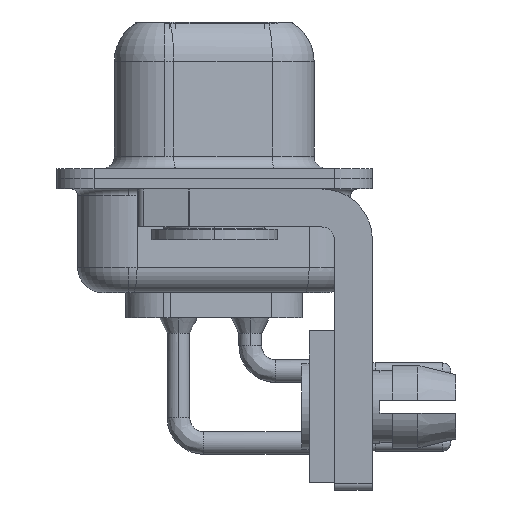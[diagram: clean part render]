
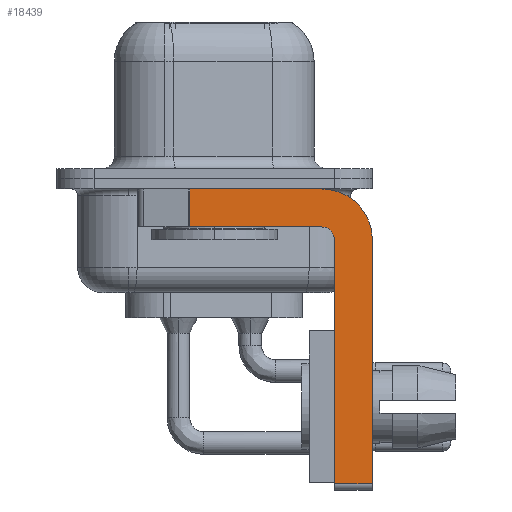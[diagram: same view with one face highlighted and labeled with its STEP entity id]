
A CAD part, left-side view. The second image highlights one B-rep face of the part: STEP entity #18439.
In plain terms, the highlighted planar face has unit normal (-1, 0, 0).
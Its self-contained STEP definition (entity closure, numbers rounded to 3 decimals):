
#227 = EDGE_LOOP ( 'NONE', ( #13423, #16876, #19151, #14804, #31102, #12259, #10388, #13263 ) ) ;
#1313 = LINE ( 'NONE', #20299, #27001 ) ;
#1387 = EDGE_CURVE ( 'NONE', #9785, #28108, #3314, .T. ) ;
#2059 = LINE ( 'NONE', #22127, #14434 ) ;
#2197 = VERTEX_POINT ( 'NONE', #12103 ) ;
#3314 = CIRCLE ( 'NONE', #14173, 2. ) ;
#3638 = VERTEX_POINT ( 'NONE', #23678 ) ;
#3837 = LINE ( 'NONE', #17102, #9616 ) ;
#4691 = DIRECTION ( 'NONE',  ( 0., 0., 1. ) ) ;
#5693 = CARTESIAN_POINT ( 'NONE',  ( -2.9, -4.75, -2.4 ) ) ;
#6016 = DIRECTION ( 'NONE',  ( 0., 0., -1. ) ) ;
#7905 = EDGE_CURVE ( 'NONE', #11101, #25925, #14828, .T. ) ;
#8450 = VECTOR ( 'NONE', #6016, 1000. ) ;
#8511 = VECTOR ( 'NONE', #18971, 1000. ) ;
#8834 = AXIS2_PLACEMENT_3D ( 'NONE', #12398, #29939, #14908 ) ;
#9466 = EDGE_CURVE ( 'NONE', #22974, #2197, #21409, .T. ) ;
#9616 = VECTOR ( 'NONE', #4691, 1000. ) ;
#9785 = VERTEX_POINT ( 'NONE', #25731 ) ;
#10388 = ORIENTED_EDGE ( 'NONE', *, *, #11176, .F. ) ;
#11101 = VERTEX_POINT ( 'NONE', #5693 ) ;
#11176 = EDGE_CURVE ( 'NONE', #28108, #3638, #20982, .T. ) ;
#11508 = CARTESIAN_POINT ( 'NONE',  ( -2.9, -4.25, -12.05 ) ) ;
#12103 = CARTESIAN_POINT ( 'NONE',  ( -2.9, 0.978, -1.9 ) ) ;
#12259 = ORIENTED_EDGE ( 'NONE', *, *, #15803, .T. ) ;
#12398 = CARTESIAN_POINT ( 'NONE',  ( -2.9, -4.25, -2.4 ) ) ;
#12971 = CARTESIAN_POINT ( 'NONE',  ( -2.9, -4.25, -2.4 ) ) ;
#13248 = CARTESIAN_POINT ( 'NONE',  ( -2.9, -4.75, -12.05 ) ) ;
#13263 = ORIENTED_EDGE ( 'NONE', *, *, #1387, .F. ) ;
#13423 = ORIENTED_EDGE ( 'NONE', *, *, #22481, .F. ) ;
#13800 = DIRECTION ( 'NONE',  ( 0., 0., -1. ) ) ;
#14131 = EDGE_CURVE ( 'NONE', #25925, #2197, #1313, .T. ) ;
#14173 = AXIS2_PLACEMENT_3D ( 'NONE', #14402, #14373, #13800 ) ;
#14371 = LINE ( 'NONE', #11508, #8511 ) ;
#14373 = DIRECTION ( 'NONE',  ( 1., 0., 0. ) ) ;
#14402 = CARTESIAN_POINT ( 'NONE',  ( -2.9, -4.25, -2.4 ) ) ;
#14434 = VECTOR ( 'NONE', #22235, 1000. ) ;
#14736 = VECTOR ( 'NONE', #24557, 1000. ) ;
#14804 = ORIENTED_EDGE ( 'NONE', *, *, #7905, .F. ) ;
#14828 = CIRCLE ( 'NONE', #20042, 0.5 ) ;
#14908 = DIRECTION ( 'NONE',  ( 0., 0., -1. ) ) ;
#15203 = CARTESIAN_POINT ( 'NONE',  ( -2.9, -6.25, -2.4 ) ) ;
#15358 = DIRECTION ( 'NONE',  ( 0., 1., 0. ) ) ;
#15482 = DIRECTION ( 'NONE',  ( 0., 0., 1. ) ) ;
#15803 = EDGE_CURVE ( 'NONE', #31345, #3638, #14371, .T. ) ;
#16876 = ORIENTED_EDGE ( 'NONE', *, *, #9466, .T. ) ;
#17018 = CARTESIAN_POINT ( 'NONE',  ( -2.9, 0.978, -1.9 ) ) ;
#17102 = CARTESIAN_POINT ( 'NONE',  ( -2.9, -4.75, -12.3 ) ) ;
#18439 = ADVANCED_FACE ( 'NONE', ( #31940 ), #27383, .F. ) ;
#18971 = DIRECTION ( 'NONE',  ( 0., -1., 0. ) ) ;
#19151 = ORIENTED_EDGE ( 'NONE', *, *, #14131, .F. ) ;
#20042 = AXIS2_PLACEMENT_3D ( 'NONE', #12971, #30501, #15482 ) ;
#20299 = CARTESIAN_POINT ( 'NONE',  ( -2.9, -4.25, -1.9 ) ) ;
#20962 = CARTESIAN_POINT ( 'NONE',  ( -2.9, -6.25, -2.4 ) ) ;
#20982 = LINE ( 'NONE', #20962, #8450 ) ;
#21409 = LINE ( 'NONE', #17018, #14736 ) ;
#22127 = CARTESIAN_POINT ( 'NONE',  ( -2.9, 3., -0.4 ) ) ;
#22235 = DIRECTION ( 'NONE',  ( 0., -1., 0. ) ) ;
#22481 = EDGE_CURVE ( 'NONE', #22974, #9785, #2059, .T. ) ;
#22974 = VERTEX_POINT ( 'NONE', #29527 ) ;
#23678 = CARTESIAN_POINT ( 'NONE',  ( -2.9, -6.25, -12.05 ) ) ;
#23728 = CARTESIAN_POINT ( 'NONE',  ( -2.9, -4.25, -1.9 ) ) ;
#24557 = DIRECTION ( 'NONE',  ( 0., 0., -1. ) ) ;
#24621 = EDGE_CURVE ( 'NONE', #31345, #11101, #3837, .T. ) ;
#25731 = CARTESIAN_POINT ( 'NONE',  ( -2.9, -4.25, -0.4 ) ) ;
#25925 = VERTEX_POINT ( 'NONE', #23728 ) ;
#27001 = VECTOR ( 'NONE', #15358, 1000. ) ;
#27383 = PLANE ( 'NONE',  #8834 ) ;
#28108 = VERTEX_POINT ( 'NONE', #15203 ) ;
#29527 = CARTESIAN_POINT ( 'NONE',  ( -2.9, 0.978, -0.4 ) ) ;
#29939 = DIRECTION ( 'NONE',  ( 1., 0., 0. ) ) ;
#30501 = DIRECTION ( 'NONE',  ( -1., 0., 0. ) ) ;
#31102 = ORIENTED_EDGE ( 'NONE', *, *, #24621, .F. ) ;
#31345 = VERTEX_POINT ( 'NONE', #13248 ) ;
#31940 = FACE_OUTER_BOUND ( 'NONE', #227, .T. ) ;
